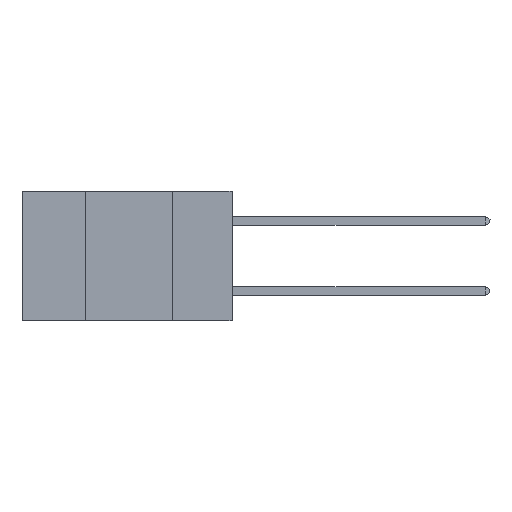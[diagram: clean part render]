
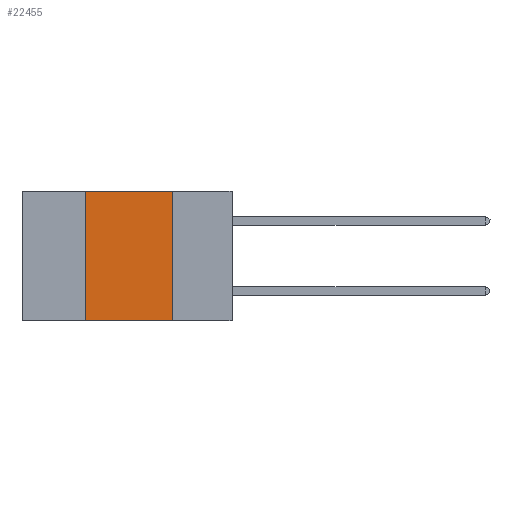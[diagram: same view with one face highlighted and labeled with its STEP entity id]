
A CAD part, left-side view. The second image highlights one B-rep face of the part: STEP entity #22455.
In plain terms, the highlighted planar face has unit normal (-1, 0, 0).
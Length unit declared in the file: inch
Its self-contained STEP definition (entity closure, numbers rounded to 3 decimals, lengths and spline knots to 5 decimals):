
#470 = ORIENTED_EDGE ( 'NONE', *, *, #9193, .T. ) ;
#2209 = VERTEX_POINT ( 'NONE', #6694 ) ;
#2415 = EDGE_LOOP ( 'NONE', ( #7327, #24925, #12126, #470 ) ) ;
#2462 = CARTESIAN_POINT ( 'NONE',  ( 0., 0.17, 0. ) ) ;
#2758 = CARTESIAN_POINT ( 'NONE',  ( 0., 0.6, 0. ) ) ;
#3132 = DIRECTION ( 'NONE',  ( 0., 0., 1. ) ) ;
#3703 = FACE_OUTER_BOUND ( 'NONE', #2415, .T. ) ;
#3886 = CARTESIAN_POINT ( 'NONE',  ( 0., 0.17, -0.37 ) ) ;
#4848 = PLANE ( 'NONE',  #8928 ) ;
#5049 = EDGE_CURVE ( 'NONE', #2209, #15790, #15652, .T. ) ;
#5273 = VERTEX_POINT ( 'NONE', #2462 ) ;
#6694 = CARTESIAN_POINT ( 'NONE',  ( 0., 0.42, -0.37 ) ) ;
#7327 = ORIENTED_EDGE ( 'NONE', *, *, #27363, .F. ) ;
#8928 = AXIS2_PLACEMENT_3D ( 'NONE', #2758, #9073, #11111 ) ;
#9073 = DIRECTION ( 'NONE',  ( 1., 0., 0. ) ) ;
#9193 = EDGE_CURVE ( 'NONE', #2209, #24088, #16475, .T. ) ;
#10273 = CARTESIAN_POINT ( 'NONE',  ( 0., 0.42, 0. ) ) ;
#10470 = DIRECTION ( 'NONE',  ( 0., -1., 0. ) ) ;
#10778 = VECTOR ( 'NONE', #23816, 39.37008 ) ;
#11111 = DIRECTION ( 'NONE',  ( 0., 0., -1. ) ) ;
#12126 = ORIENTED_EDGE ( 'NONE', *, *, #5049, .F. ) ;
#12266 = VECTOR ( 'NONE', #10470, 39.37008 ) ;
#12575 = CARTESIAN_POINT ( 'NONE',  ( 0., 0.17, 0. ) ) ;
#15259 = CARTESIAN_POINT ( 'NONE',  ( 0., 0.6, -0.37 ) ) ;
#15652 = LINE ( 'NONE', #15965, #16330 ) ;
#15790 = VERTEX_POINT ( 'NONE', #10273 ) ;
#15965 = CARTESIAN_POINT ( 'NONE',  ( 0., 0.42, 0. ) ) ;
#16330 = VECTOR ( 'NONE', #3132, 39.37008 ) ;
#16475 = LINE ( 'NONE', #15259, #10778 ) ;
#17152 = LINE ( 'NONE', #12575, #26513 ) ;
#17710 = EDGE_CURVE ( 'NONE', #15790, #5273, #19923, .T. ) ;
#19923 = LINE ( 'NONE', #25742, #12266 ) ;
#22455 = ADVANCED_FACE ( 'NONE', ( #3703 ), #4848, .F. ) ;
#22459 = DIRECTION ( 'NONE',  ( 0., 0., -1. ) ) ;
#23816 = DIRECTION ( 'NONE',  ( 0., -1., 0. ) ) ;
#24088 = VERTEX_POINT ( 'NONE', #3886 ) ;
#24925 = ORIENTED_EDGE ( 'NONE', *, *, #17710, .F. ) ;
#25742 = CARTESIAN_POINT ( 'NONE',  ( 0., 0.6, 0. ) ) ;
#26513 = VECTOR ( 'NONE', #22459, 39.37008 ) ;
#27363 = EDGE_CURVE ( 'NONE', #5273, #24088, #17152, .T. ) ;
